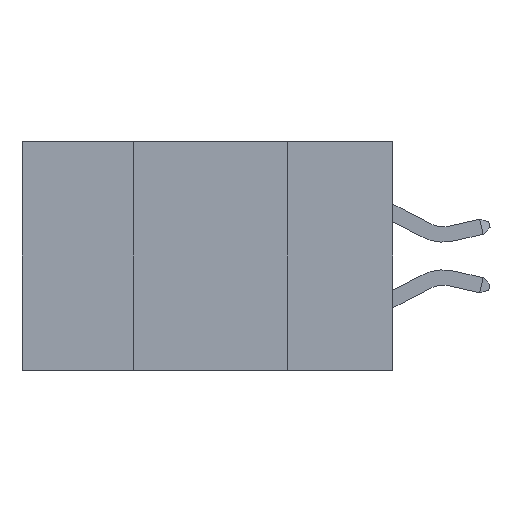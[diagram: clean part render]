
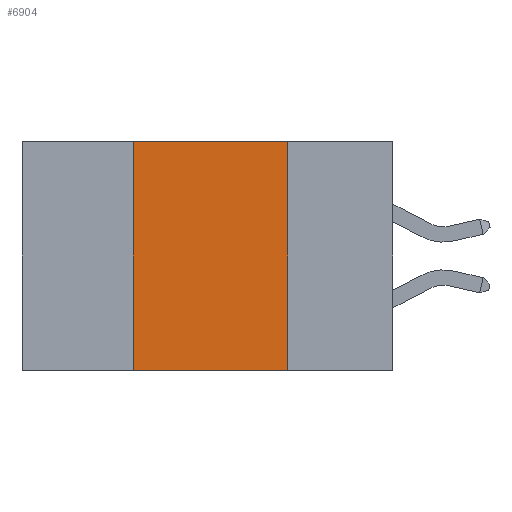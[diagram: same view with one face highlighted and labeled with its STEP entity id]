
A CAD part, left-side view. The second image highlights one B-rep face of the part: STEP entity #6904.
In plain terms, the highlighted planar face has unit normal (-1, 0, 0).
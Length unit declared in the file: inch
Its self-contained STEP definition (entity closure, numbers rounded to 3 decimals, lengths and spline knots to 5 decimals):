
#72 = PLANE ( 'NONE',  #15364 ) ;
#78 = EDGE_CURVE ( 'NONE', #14708, #12963, #15216, .T. ) ;
#1084 = ORIENTED_EDGE ( 'NONE', *, *, #20240, .F. ) ;
#2063 = EDGE_LOOP ( 'NONE', ( #8708, #13927, #1084, #5935 ) ) ;
#2997 = CARTESIAN_POINT ( 'NONE',  ( 0., 0.42, 0. ) ) ;
#3087 = VERTEX_POINT ( 'NONE', #2997 ) ;
#3624 = VECTOR ( 'NONE', #9501, 39.37008 ) ;
#4501 = VECTOR ( 'NONE', #11211, 39.37008 ) ;
#4742 = EDGE_CURVE ( 'NONE', #3087, #9712, #19328, .T. ) ;
#5071 = DIRECTION ( 'NONE',  ( 0., 0., -1. ) ) ;
#5266 = CARTESIAN_POINT ( 'NONE',  ( 0., 0.17, 0. ) ) ;
#5935 = ORIENTED_EDGE ( 'NONE', *, *, #78, .T. ) ;
#6694 = CARTESIAN_POINT ( 'NONE',  ( 0., 0.6, 0. ) ) ;
#6904 = ADVANCED_FACE ( 'NONE', ( #7012 ), #72, .F. ) ;
#7012 = FACE_OUTER_BOUND ( 'NONE', #2063, .T. ) ;
#7020 = LINE ( 'NONE', #7128, #12386 ) ;
#7128 = CARTESIAN_POINT ( 'NONE',  ( 0., 0.17, 0. ) ) ;
#7777 = CARTESIAN_POINT ( 'NONE',  ( 0., 0.42, 0. ) ) ;
#8708 = ORIENTED_EDGE ( 'NONE', *, *, #13309, .F. ) ;
#9151 = VECTOR ( 'NONE', #15107, 39.37008 ) ;
#9501 = DIRECTION ( 'NONE',  ( 0., -1., 0. ) ) ;
#9712 = VERTEX_POINT ( 'NONE', #5266 ) ;
#10671 = CARTESIAN_POINT ( 'NONE',  ( 0., 0.6, -0.37 ) ) ;
#11211 = DIRECTION ( 'NONE',  ( 0., 0., 1. ) ) ;
#12386 = VECTOR ( 'NONE', #15027, 39.37008 ) ;
#12941 = LINE ( 'NONE', #7777, #4501 ) ;
#12963 = VERTEX_POINT ( 'NONE', #16977 ) ;
#13309 = EDGE_CURVE ( 'NONE', #9712, #12963, #7020, .T. ) ;
#13400 = CARTESIAN_POINT ( 'NONE',  ( 0., 0.42, -0.37 ) ) ;
#13927 = ORIENTED_EDGE ( 'NONE', *, *, #4742, .F. ) ;
#14708 = VERTEX_POINT ( 'NONE', #13400 ) ;
#15027 = DIRECTION ( 'NONE',  ( 0., 0., -1. ) ) ;
#15107 = DIRECTION ( 'NONE',  ( 0., -1., 0. ) ) ;
#15216 = LINE ( 'NONE', #10671, #9151 ) ;
#15364 = AXIS2_PLACEMENT_3D ( 'NONE', #6694, #19894, #5071 ) ;
#15765 = CARTESIAN_POINT ( 'NONE',  ( 0., 0.6, 0. ) ) ;
#16977 = CARTESIAN_POINT ( 'NONE',  ( 0., 0.17, -0.37 ) ) ;
#19328 = LINE ( 'NONE', #15765, #3624 ) ;
#19894 = DIRECTION ( 'NONE',  ( 1., 0., 0. ) ) ;
#20240 = EDGE_CURVE ( 'NONE', #14708, #3087, #12941, .T. ) ;
